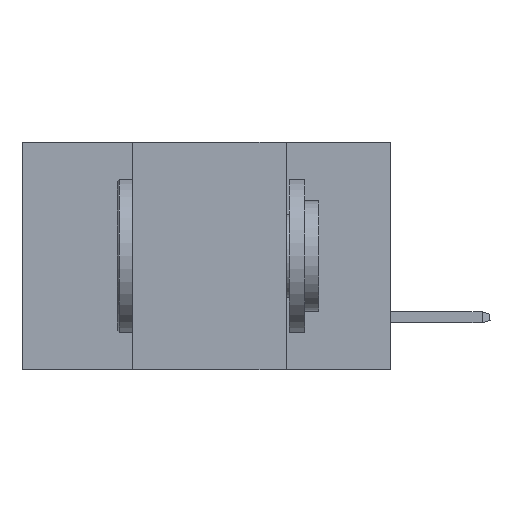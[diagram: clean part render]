
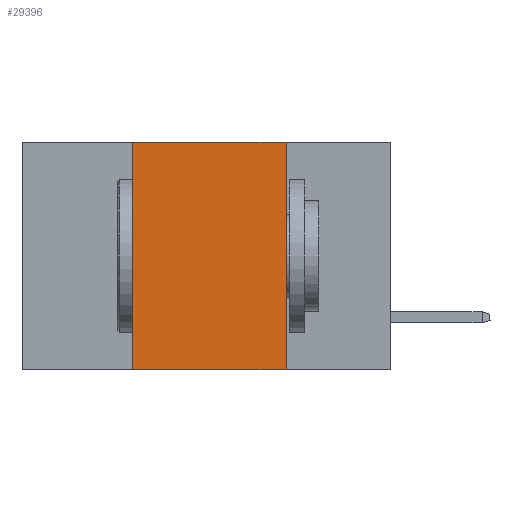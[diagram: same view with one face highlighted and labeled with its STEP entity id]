
A CAD part, left-side view. The second image highlights one B-rep face of the part: STEP entity #29396.
In plain terms, the highlighted planar face has unit normal (-1, 0, 0).
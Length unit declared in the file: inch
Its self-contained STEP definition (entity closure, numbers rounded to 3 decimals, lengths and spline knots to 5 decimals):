
#22 = EDGE_CURVE ( 'NONE', #32574, #12098, #30083, .T. ) ;
#314 = CARTESIAN_POINT ( 'NONE',  ( 0., 0.17, 0. ) ) ;
#597 = EDGE_LOOP ( 'NONE', ( #25778, #1924, #34315, #19677 ) ) ;
#1191 = CARTESIAN_POINT ( 'NONE',  ( 0., 0.42, 0. ) ) ;
#1924 = ORIENTED_EDGE ( 'NONE', *, *, #23582, .F. ) ;
#1935 = EDGE_CURVE ( 'NONE', #32574, #27909, #9222, .T. ) ;
#1991 = CARTESIAN_POINT ( 'NONE',  ( 0., 0.17, 0. ) ) ;
#3286 = VECTOR ( 'NONE', #23741, 39.37008 ) ;
#3461 = CARTESIAN_POINT ( 'NONE',  ( 0., 0.42, -0.37 ) ) ;
#6543 = VERTEX_POINT ( 'NONE', #314 ) ;
#6746 = DIRECTION ( 'NONE',  ( 0., -1., 0. ) ) ;
#6866 = CARTESIAN_POINT ( 'NONE',  ( 0., 0.6, 0. ) ) ;
#7510 = DIRECTION ( 'NONE',  ( 0., -1., 0. ) ) ;
#9222 = LINE ( 'NONE', #33791, #15447 ) ;
#10095 = DIRECTION ( 'NONE',  ( 1., 0., 0. ) ) ;
#12098 = VERTEX_POINT ( 'NONE', #15915 ) ;
#12738 = DIRECTION ( 'NONE',  ( 0., 0., -1. ) ) ;
#15447 = VECTOR ( 'NONE', #28136, 39.37008 ) ;
#15545 = LINE ( 'NONE', #1991, #3286 ) ;
#15831 = EDGE_CURVE ( 'NONE', #6543, #12098, #15545, .T. ) ;
#15915 = CARTESIAN_POINT ( 'NONE',  ( 0., 0.17, -0.37 ) ) ;
#17836 = CARTESIAN_POINT ( 'NONE',  ( 0., 0.6, 0. ) ) ;
#19677 = ORIENTED_EDGE ( 'NONE', *, *, #22, .T. ) ;
#20121 = VECTOR ( 'NONE', #6746, 39.37008 ) ;
#23582 = EDGE_CURVE ( 'NONE', #27909, #6543, #30524, .T. ) ;
#23741 = DIRECTION ( 'NONE',  ( 0., 0., -1. ) ) ;
#25778 = ORIENTED_EDGE ( 'NONE', *, *, #15831, .F. ) ;
#27909 = VERTEX_POINT ( 'NONE', #1191 ) ;
#28136 = DIRECTION ( 'NONE',  ( 0., 0., 1. ) ) ;
#28273 = CARTESIAN_POINT ( 'NONE',  ( 0., 0.6, -0.37 ) ) ;
#29396 = ADVANCED_FACE ( 'NONE', ( #34064 ), #33765, .F. ) ;
#30083 = LINE ( 'NONE', #28273, #30924 ) ;
#30524 = LINE ( 'NONE', #6866, #20121 ) ;
#30924 = VECTOR ( 'NONE', #7510, 39.37008 ) ;
#32400 = AXIS2_PLACEMENT_3D ( 'NONE', #17836, #10095, #12738 ) ;
#32574 = VERTEX_POINT ( 'NONE', #3461 ) ;
#33765 = PLANE ( 'NONE',  #32400 ) ;
#33791 = CARTESIAN_POINT ( 'NONE',  ( 0., 0.42, 0. ) ) ;
#34064 = FACE_OUTER_BOUND ( 'NONE', #597, .T. ) ;
#34315 = ORIENTED_EDGE ( 'NONE', *, *, #1935, .F. ) ;
